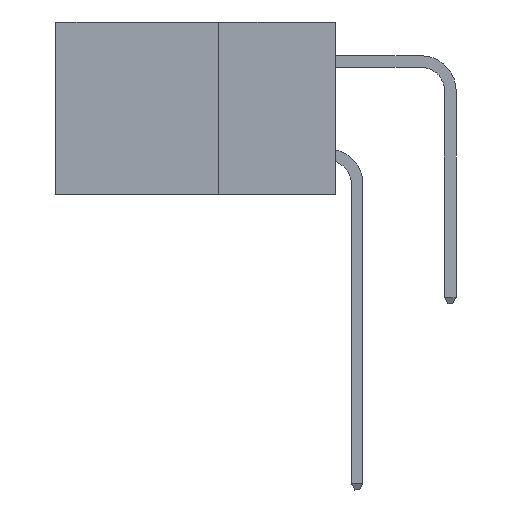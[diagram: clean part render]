
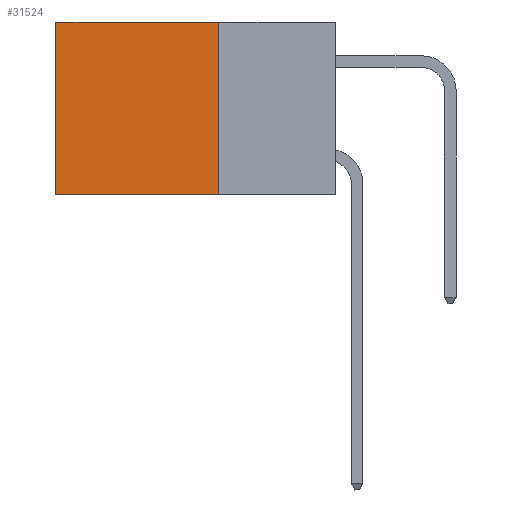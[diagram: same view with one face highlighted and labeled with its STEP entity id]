
A CAD part, left-side view. The second image highlights one B-rep face of the part: STEP entity #31524.
In plain terms, the highlighted planar face has unit normal (-1, 0, 0).
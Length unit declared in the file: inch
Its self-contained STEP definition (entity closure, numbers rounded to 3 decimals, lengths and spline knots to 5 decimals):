
#2019 = CARTESIAN_POINT ( 'NONE',  ( 0.2875, 0.25, -0.37 ) ) ;
#2350 = ORIENTED_EDGE ( 'NONE', *, *, #15851, .F. ) ;
#2842 = CARTESIAN_POINT ( 'NONE',  ( 0.2875, 0.25, 0. ) ) ;
#3976 = CARTESIAN_POINT ( 'NONE',  ( 0.2875, 0.6, 0. ) ) ;
#4201 = LINE ( 'NONE', #28168, #33415 ) ;
#5476 = ORIENTED_EDGE ( 'NONE', *, *, #7108, .T. ) ;
#5574 = LINE ( 'NONE', #28657, #19985 ) ;
#6406 = VERTEX_POINT ( 'NONE', #2019 ) ;
#6417 = EDGE_CURVE ( 'NONE', #15249, #6406, #34757, .T. ) ;
#6633 = EDGE_CURVE ( 'NONE', #15890, #14115, #5574, .T. ) ;
#7108 = EDGE_CURVE ( 'NONE', #15249, #15890, #4201, .T. ) ;
#7575 = FACE_OUTER_BOUND ( 'NONE', #18939, .T. ) ;
#14115 = VERTEX_POINT ( 'NONE', #27888 ) ;
#15249 = VERTEX_POINT ( 'NONE', #24693 ) ;
#15851 = EDGE_CURVE ( 'NONE', #6406, #14115, #33236, .T. ) ;
#15890 = VERTEX_POINT ( 'NONE', #3976 ) ;
#18939 = EDGE_LOOP ( 'NONE', ( #29230, #2350, #25992, #5476 ) ) ;
#19985 = VECTOR ( 'NONE', #25883, 39.37008 ) ;
#22239 = DIRECTION ( 'NONE',  ( 0., 1., 0. ) ) ;
#24693 = CARTESIAN_POINT ( 'NONE',  ( 0.2875, 0.25, 0. ) ) ;
#24871 = CARTESIAN_POINT ( 'NONE',  ( 0.2875, 0.25, 0. ) ) ;
#25644 = VECTOR ( 'NONE', #36304, 39.37008 ) ;
#25883 = DIRECTION ( 'NONE',  ( 0., 0., -1. ) ) ;
#25908 = DIRECTION ( 'NONE',  ( 1., 0., 0. ) ) ;
#25992 = ORIENTED_EDGE ( 'NONE', *, *, #6417, .F. ) ;
#27239 = VECTOR ( 'NONE', #36847, 39.37008 ) ;
#27888 = CARTESIAN_POINT ( 'NONE',  ( 0.2875, 0.6, -0.37 ) ) ;
#28168 = CARTESIAN_POINT ( 'NONE',  ( 0.2875, 0.25, 0. ) ) ;
#28657 = CARTESIAN_POINT ( 'NONE',  ( 0.2875, 0.6, 0. ) ) ;
#28796 = DIRECTION ( 'NONE',  ( 0., 0., -1. ) ) ;
#29230 = ORIENTED_EDGE ( 'NONE', *, *, #6633, .T. ) ;
#30263 = AXIS2_PLACEMENT_3D ( 'NONE', #2842, #25908, #28796 ) ;
#30828 = CARTESIAN_POINT ( 'NONE',  ( 0.2875, 0.25, -0.37 ) ) ;
#31524 = ADVANCED_FACE ( 'NONE', ( #7575 ), #34147, .F. ) ;
#33236 = LINE ( 'NONE', #30828, #25644 ) ;
#33415 = VECTOR ( 'NONE', #22239, 39.37008 ) ;
#34147 = PLANE ( 'NONE',  #30263 ) ;
#34757 = LINE ( 'NONE', #24871, #27239 ) ;
#36304 = DIRECTION ( 'NONE',  ( 0., 1., 0. ) ) ;
#36847 = DIRECTION ( 'NONE',  ( 0., 0., -1. ) ) ;
